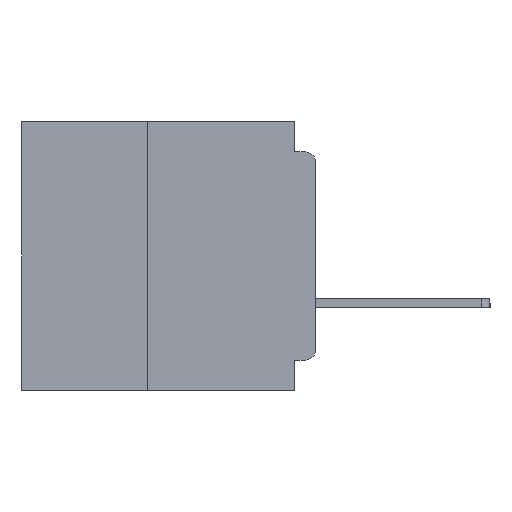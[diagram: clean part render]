
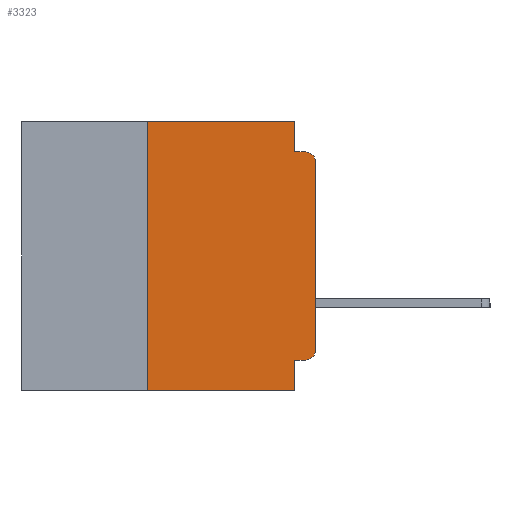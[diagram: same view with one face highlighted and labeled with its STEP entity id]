
A CAD part, left-side view. The second image highlights one B-rep face of the part: STEP entity #3323.
In plain terms, the highlighted planar face has unit normal (-1, 0, 0).
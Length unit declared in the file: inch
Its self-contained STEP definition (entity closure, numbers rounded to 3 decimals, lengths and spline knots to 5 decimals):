
#1192 = ORIENTED_EDGE ( 'NONE', *, *, #29301, .T. ) ;
#2022 = ORIENTED_EDGE ( 'NONE', *, *, #30097, .T. ) ;
#2300 = PLANE ( 'NONE',  #31785 ) ;
#2367 = DIRECTION ( 'NONE',  ( 0., 0., -1. ) ) ;
#2796 = DIRECTION ( 'NONE',  ( 0., -1., 0. ) ) ;
#3295 = AXIS2_PLACEMENT_3D ( 'NONE', #40484, #21469, #2367 ) ;
#3304 = CARTESIAN_POINT ( 'NONE',  ( 0., 0.015, -0.34 ) ) ;
#3323 = ADVANCED_FACE ( 'NONE', ( #7167 ), #2300, .F. ) ;
#5527 = DIRECTION ( 'NONE',  ( 1., 0., 0. ) ) ;
#5742 = CARTESIAN_POINT ( 'NONE',  ( 0., 0.031, 0. ) ) ;
#6156 = VECTOR ( 'NONE', #8958, 39.37008 ) ;
#6492 = DIRECTION ( 'NONE',  ( 0., 0., -1. ) ) ;
#7167 = FACE_OUTER_BOUND ( 'NONE', #18581, .T. ) ;
#7673 = CARTESIAN_POINT ( 'NONE',  ( 0., 0.031, -0.045 ) ) ;
#7952 = VERTEX_POINT ( 'NONE', #16342 ) ;
#8160 = ORIENTED_EDGE ( 'NONE', *, *, #24712, .F. ) ;
#8733 = VERTEX_POINT ( 'NONE', #7673 ) ;
#8958 = DIRECTION ( 'NONE',  ( 0., 0., -1. ) ) ;
#9374 = AXIS2_PLACEMENT_3D ( 'NONE', #3304, #25529, #6492 ) ;
#9852 = ORIENTED_EDGE ( 'NONE', *, *, #12187, .F. ) ;
#10546 = EDGE_CURVE ( 'NONE', #15502, #40043, #21216, .T. ) ;
#10709 = CARTESIAN_POINT ( 'NONE',  ( 0., 0., -0.06 ) ) ;
#11564 = VERTEX_POINT ( 'NONE', #17328 ) ;
#12125 = VERTEX_POINT ( 'NONE', #10709 ) ;
#12187 = EDGE_CURVE ( 'NONE', #8733, #21182, #14568, .T. ) ;
#12975 = VECTOR ( 'NONE', #21423, 39.37008 ) ;
#13326 = ORIENTED_EDGE ( 'NONE', *, *, #26837, .T. ) ;
#13489 = DIRECTION ( 'NONE',  ( 0., 0., -1. ) ) ;
#14148 = CARTESIAN_POINT ( 'NONE',  ( 0., 0., 0. ) ) ;
#14209 = CARTESIAN_POINT ( 'NONE',  ( 0., 0., -0.045 ) ) ;
#14568 = LINE ( 'NONE', #14209, #30505 ) ;
#14793 = CARTESIAN_POINT ( 'NONE',  ( 0., 0.031, -0.4 ) ) ;
#15502 = VERTEX_POINT ( 'NONE', #23372 ) ;
#16342 = CARTESIAN_POINT ( 'NONE',  ( 0., 0.031, -0.355 ) ) ;
#17328 = CARTESIAN_POINT ( 'NONE',  ( 0., 0.015, -0.355 ) ) ;
#17422 = DIRECTION ( 'NONE',  ( 0., -1., 0. ) ) ;
#17814 = CIRCLE ( 'NONE', #3295, 0.015 ) ;
#18462 = ORIENTED_EDGE ( 'NONE', *, *, #35394, .F. ) ;
#18581 = EDGE_LOOP ( 'NONE', ( #1192, #2022, #9852, #18462, #37667, #36981, #13326, #8160, #22198, #31287 ) ) ;
#19208 = LINE ( 'NONE', #31406, #35126 ) ;
#19441 = EDGE_CURVE ( 'NONE', #11564, #40721, #27837, .T. ) ;
#20150 = LINE ( 'NONE', #23108, #37036 ) ;
#21182 = VERTEX_POINT ( 'NONE', #25262 ) ;
#21216 = LINE ( 'NONE', #40867, #37105 ) ;
#21398 = CARTESIAN_POINT ( 'NONE',  ( 0., 0.437, 0. ) ) ;
#21423 = DIRECTION ( 'NONE',  ( 0., 1., 0. ) ) ;
#21469 = DIRECTION ( 'NONE',  ( -1., 0., 0. ) ) ;
#22198 = ORIENTED_EDGE ( 'NONE', *, *, #36504, .F. ) ;
#22418 = CARTESIAN_POINT ( 'NONE',  ( 0., 0.437, -0.4 ) ) ;
#23108 = CARTESIAN_POINT ( 'NONE',  ( 0., 0.031, -0.4 ) ) ;
#23372 = CARTESIAN_POINT ( 'NONE',  ( 0., 0.25, 0. ) ) ;
#24712 = EDGE_CURVE ( 'NONE', #7952, #39123, #20150, .T. ) ;
#24756 = VECTOR ( 'NONE', #39596, 39.37008 ) ;
#25025 = LINE ( 'NONE', #22418, #40935 ) ;
#25262 = CARTESIAN_POINT ( 'NONE',  ( 0., 0.015, -0.045 ) ) ;
#25529 = DIRECTION ( 'NONE',  ( -1., 0., 0. ) ) ;
#26117 = CARTESIAN_POINT ( 'NONE',  ( 0., 0.031, 0. ) ) ;
#26837 = EDGE_CURVE ( 'NONE', #28728, #39123, #25025, .T. ) ;
#27767 = DIRECTION ( 'NONE',  ( 0., 0., -1. ) ) ;
#27837 = CIRCLE ( 'NONE', #9374, 0.015 ) ;
#28728 = VERTEX_POINT ( 'NONE', #30204 ) ;
#28796 = DIRECTION ( 'NONE',  ( 0., -1., 0. ) ) ;
#29301 = EDGE_CURVE ( 'NONE', #40721, #12125, #33227, .T. ) ;
#30097 = EDGE_CURVE ( 'NONE', #12125, #21182, #17814, .T. ) ;
#30204 = CARTESIAN_POINT ( 'NONE',  ( 0., 0.25, -0.4 ) ) ;
#30505 = VECTOR ( 'NONE', #17422, 39.37008 ) ;
#30864 = CARTESIAN_POINT ( 'NONE',  ( 0., 0., -0.355 ) ) ;
#30923 = LINE ( 'NONE', #30864, #12975 ) ;
#31102 = EDGE_CURVE ( 'NONE', #28728, #15502, #19208, .T. ) ;
#31287 = ORIENTED_EDGE ( 'NONE', *, *, #19441, .T. ) ;
#31406 = CARTESIAN_POINT ( 'NONE',  ( 0., 0.25, -0.4 ) ) ;
#31519 = LINE ( 'NONE', #5742, #6156 ) ;
#31785 = AXIS2_PLACEMENT_3D ( 'NONE', #21398, #5527, #27767 ) ;
#33227 = LINE ( 'NONE', #14148, #24756 ) ;
#34625 = DIRECTION ( 'NONE',  ( 0., 0., 1. ) ) ;
#35126 = VECTOR ( 'NONE', #34625, 39.37008 ) ;
#35394 = EDGE_CURVE ( 'NONE', #40043, #8733, #31519, .T. ) ;
#36093 = CARTESIAN_POINT ( 'NONE',  ( 0., 0., -0.34 ) ) ;
#36504 = EDGE_CURVE ( 'NONE', #11564, #7952, #30923, .T. ) ;
#36981 = ORIENTED_EDGE ( 'NONE', *, *, #31102, .F. ) ;
#37036 = VECTOR ( 'NONE', #13489, 39.37008 ) ;
#37105 = VECTOR ( 'NONE', #2796, 39.37008 ) ;
#37667 = ORIENTED_EDGE ( 'NONE', *, *, #10546, .F. ) ;
#39123 = VERTEX_POINT ( 'NONE', #14793 ) ;
#39596 = DIRECTION ( 'NONE',  ( 0., 0., 1. ) ) ;
#40043 = VERTEX_POINT ( 'NONE', #26117 ) ;
#40484 = CARTESIAN_POINT ( 'NONE',  ( 0., 0.015, -0.06 ) ) ;
#40721 = VERTEX_POINT ( 'NONE', #36093 ) ;
#40867 = CARTESIAN_POINT ( 'NONE',  ( 0., 0.437, 0. ) ) ;
#40935 = VECTOR ( 'NONE', #28796, 39.37008 ) ;
